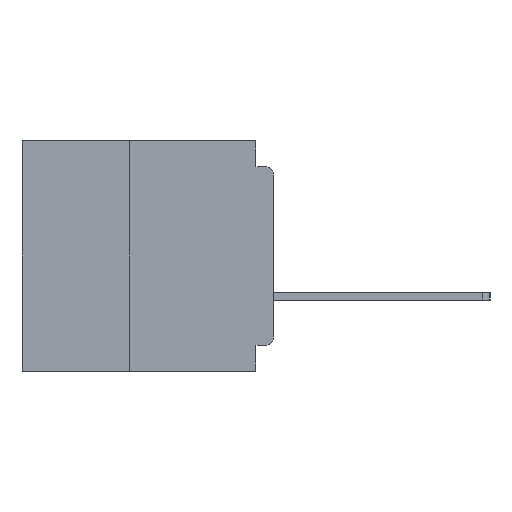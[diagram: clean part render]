
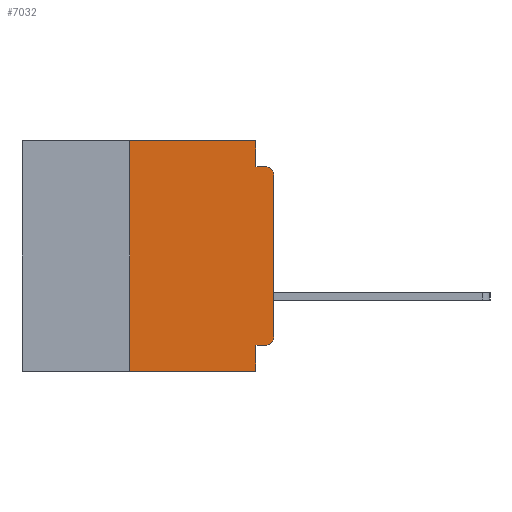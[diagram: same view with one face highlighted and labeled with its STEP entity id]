
A CAD part, left-side view. The second image highlights one B-rep face of the part: STEP entity #7032.
In plain terms, the highlighted planar face has unit normal (-1, 0, 0).
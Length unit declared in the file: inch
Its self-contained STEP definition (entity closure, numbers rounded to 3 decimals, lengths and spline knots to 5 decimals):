
#1200 = ORIENTED_EDGE ( 'NONE', *, *, #33128, .T. ) ;
#1281 = PLANE ( 'NONE',  #32323 ) ;
#1584 = VERTEX_POINT ( 'NONE', #3735 ) ;
#1921 = EDGE_CURVE ( 'NONE', #4819, #12269, #29715, .T. ) ;
#2295 = EDGE_LOOP ( 'NONE', ( #6702, #1200, #13930, #28681, #37789, #14264, #17277, #5555, #28966, #20306 ) ) ;
#2413 = CARTESIAN_POINT ( 'NONE',  ( 0., 0.015, -0.355 ) ) ;
#2766 = VERTEX_POINT ( 'NONE', #5098 ) ;
#2955 = AXIS2_PLACEMENT_3D ( 'NONE', #27862, #9852, #30860 ) ;
#3234 = VERTEX_POINT ( 'NONE', #7920 ) ;
#3446 = DIRECTION ( 'NONE',  ( -1., 0., 0. ) ) ;
#3735 = CARTESIAN_POINT ( 'NONE',  ( 0., 0.031, -0.4 ) ) ;
#3761 = VECTOR ( 'NONE', #15428, 39.37008 ) ;
#3762 = LINE ( 'NONE', #29406, #34950 ) ;
#3920 = CARTESIAN_POINT ( 'NONE',  ( 0., 0., -0.355 ) ) ;
#4819 = VERTEX_POINT ( 'NONE', #2413 ) ;
#5098 = CARTESIAN_POINT ( 'NONE',  ( 0., 0.25, -0.4 ) ) ;
#5555 = ORIENTED_EDGE ( 'NONE', *, *, #9963, .F. ) ;
#6702 = ORIENTED_EDGE ( 'NONE', *, *, #28370, .T. ) ;
#7032 = ADVANCED_FACE ( 'NONE', ( #10541 ), #1281, .F. ) ;
#7077 = VECTOR ( 'NONE', #32061, 39.37008 ) ;
#7568 = CARTESIAN_POINT ( 'NONE',  ( 0., 0.437, 0. ) ) ;
#7607 = CARTESIAN_POINT ( 'NONE',  ( 0., 0.25, -0.4 ) ) ;
#7920 = CARTESIAN_POINT ( 'NONE',  ( 0., 0.031, 0. ) ) ;
#8157 = LINE ( 'NONE', #31057, #21454 ) ;
#9696 = CIRCLE ( 'NONE', #25403, 0.015 ) ;
#9852 = DIRECTION ( 'NONE',  ( -1., 0., 0. ) ) ;
#9963 = EDGE_CURVE ( 'NONE', #12269, #1584, #8157, .T. ) ;
#10541 = FACE_OUTER_BOUND ( 'NONE', #2295, .T. ) ;
#10663 = DIRECTION ( 'NONE',  ( 0., 0., -1. ) ) ;
#11198 = EDGE_CURVE ( 'NONE', #23604, #3234, #17124, .T. ) ;
#12269 = VERTEX_POINT ( 'NONE', #12990 ) ;
#12959 = LINE ( 'NONE', #33460, #3761 ) ;
#12990 = CARTESIAN_POINT ( 'NONE',  ( 0., 0.031, -0.355 ) ) ;
#13209 = VERTEX_POINT ( 'NONE', #20723 ) ;
#13866 = VERTEX_POINT ( 'NONE', #33911 ) ;
#13930 = ORIENTED_EDGE ( 'NONE', *, *, #16364, .F. ) ;
#14264 = ORIENTED_EDGE ( 'NONE', *, *, #20138, .F. ) ;
#14732 = VECTOR ( 'NONE', #22189, 39.37008 ) ;
#14891 = CARTESIAN_POINT ( 'NONE',  ( 0., 0., -0.045 ) ) ;
#15428 = DIRECTION ( 'NONE',  ( 0., 0., -1. ) ) ;
#16364 = EDGE_CURVE ( 'NONE', #18654, #29338, #19687, .T. ) ;
#16826 = DIRECTION ( 'NONE',  ( 0., 0., 1. ) ) ;
#17120 = CARTESIAN_POINT ( 'NONE',  ( 0., 0.031, -0.045 ) ) ;
#17124 = LINE ( 'NONE', #37877, #7077 ) ;
#17277 = ORIENTED_EDGE ( 'NONE', *, *, #18109, .T. ) ;
#17936 = DIRECTION ( 'NONE',  ( 0., -1., 0. ) ) ;
#18109 = EDGE_CURVE ( 'NONE', #2766, #1584, #3762, .T. ) ;
#18654 = VERTEX_POINT ( 'NONE', #17120 ) ;
#18743 = VECTOR ( 'NONE', #17936, 39.37008 ) ;
#19687 = LINE ( 'NONE', #14891, #18743 ) ;
#20138 = EDGE_CURVE ( 'NONE', #2766, #23604, #24398, .T. ) ;
#20306 = ORIENTED_EDGE ( 'NONE', *, *, #21165, .T. ) ;
#20723 = CARTESIAN_POINT ( 'NONE',  ( 0., 0., -0.06 ) ) ;
#21165 = EDGE_CURVE ( 'NONE', #4819, #13866, #9696, .T. ) ;
#21454 = VECTOR ( 'NONE', #34056, 39.37008 ) ;
#21745 = CARTESIAN_POINT ( 'NONE',  ( 0., 0.015, -0.34 ) ) ;
#22116 = EDGE_CURVE ( 'NONE', #3234, #18654, #12959, .T. ) ;
#22189 = DIRECTION ( 'NONE',  ( 0., 1., 0. ) ) ;
#23421 = DIRECTION ( 'NONE',  ( 0., -1., 0. ) ) ;
#23604 = VERTEX_POINT ( 'NONE', #26197 ) ;
#24398 = LINE ( 'NONE', #7607, #32355 ) ;
#24706 = DIRECTION ( 'NONE',  ( 0., 0., -1. ) ) ;
#25403 = AXIS2_PLACEMENT_3D ( 'NONE', #21745, #3446, #24706 ) ;
#26197 = CARTESIAN_POINT ( 'NONE',  ( 0., 0.25, 0. ) ) ;
#27862 = CARTESIAN_POINT ( 'NONE',  ( 0., 0.015, -0.06 ) ) ;
#28349 = CIRCLE ( 'NONE', #2955, 0.015 ) ;
#28370 = EDGE_CURVE ( 'NONE', #13866, #13209, #34866, .T. ) ;
#28647 = DIRECTION ( 'NONE',  ( 1., 0., 0. ) ) ;
#28681 = ORIENTED_EDGE ( 'NONE', *, *, #22116, .F. ) ;
#28966 = ORIENTED_EDGE ( 'NONE', *, *, #1921, .F. ) ;
#29338 = VERTEX_POINT ( 'NONE', #32123 ) ;
#29406 = CARTESIAN_POINT ( 'NONE',  ( 0., 0.437, -0.4 ) ) ;
#29715 = LINE ( 'NONE', #3920, #14732 ) ;
#30860 = DIRECTION ( 'NONE',  ( 0., 0., -1. ) ) ;
#31057 = CARTESIAN_POINT ( 'NONE',  ( 0., 0.031, -0.4 ) ) ;
#32061 = DIRECTION ( 'NONE',  ( 0., -1., 0. ) ) ;
#32123 = CARTESIAN_POINT ( 'NONE',  ( 0., 0.015, -0.045 ) ) ;
#32323 = AXIS2_PLACEMENT_3D ( 'NONE', #7568, #28647, #10663 ) ;
#32355 = VECTOR ( 'NONE', #16826, 39.37008 ) ;
#33128 = EDGE_CURVE ( 'NONE', #13209, #29338, #28349, .T. ) ;
#33460 = CARTESIAN_POINT ( 'NONE',  ( 0., 0.031, 0. ) ) ;
#33911 = CARTESIAN_POINT ( 'NONE',  ( 0., 0., -0.34 ) ) ;
#33952 = VECTOR ( 'NONE', #37193, 39.37008 ) ;
#34056 = DIRECTION ( 'NONE',  ( 0., 0., -1. ) ) ;
#34238 = CARTESIAN_POINT ( 'NONE',  ( 0., 0., 0. ) ) ;
#34866 = LINE ( 'NONE', #34238, #33952 ) ;
#34950 = VECTOR ( 'NONE', #23421, 39.37008 ) ;
#37193 = DIRECTION ( 'NONE',  ( 0., 0., 1. ) ) ;
#37789 = ORIENTED_EDGE ( 'NONE', *, *, #11198, .F. ) ;
#37877 = CARTESIAN_POINT ( 'NONE',  ( 0., 0.437, 0. ) ) ;
